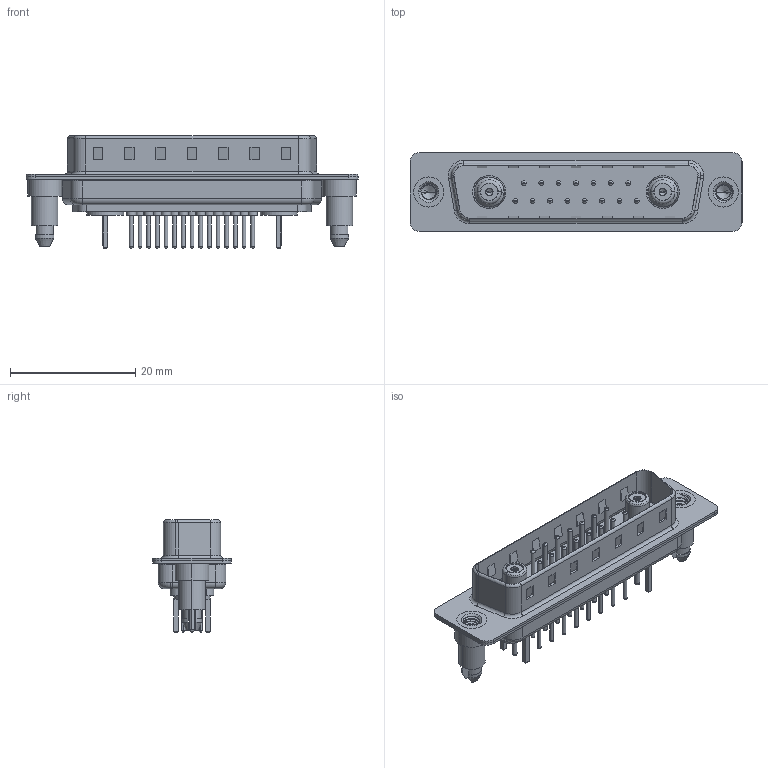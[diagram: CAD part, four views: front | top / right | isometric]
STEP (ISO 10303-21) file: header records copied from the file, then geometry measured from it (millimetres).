
FILE_DESCRIPTION (( 'STEP AP203' ), '1' );
FILE_NAME ('627-17W2224-7TD.STEP', '2019-05-27T21:48:21', ( '' ), ( '' ), 'SwSTEP 2.0', 'SolidWorks 2016', '' );
FILE_SCHEMA (( 'CONFIG_CONTROL_DESIGN' ));
Length unit declared in the file: millimetre
Products named in the file (14): Insulator Socket; 627Combo Shell Front_25 Contacts; 627Combo Threaded Boardlock_D; 627-17W2224-7TD; 627Combo Housing_17W2; Locking Collar; 627Combo Threaded Boardlock_5; 627Combo Contact Row 2_24; Co-Ax Jack Assy_S; 627Combo Contact Row 1_24; Insulator Socket 2; Co-Ax Jack_Straight PC Tail; Socket_Str; 627Combo Shell Rear_25 Contacts
Assembly tree (27 placements, depth 3):
  627-17W2224-7TD
    627Combo Housing_17W2
    627Combo Shell Rear_25 Contacts
    627Combo Shell Front_25 Contacts
    627Combo Threaded Boardlock_D
    Co-Ax Jack Assy_S  x2
      Co-Ax Jack_Straight PC Tail
      Insulator Socket
      Insulator Socket 2
      Locking Collar
      Socket_Str
    627Combo Threaded Boardlock_5
    627Combo Contact Row 1_24  x7
    627Combo Contact Row 2_24  x8
Bounding box: 53 x 12.6 x 17.9 mm (x, y, z)
Volume: 2896.4 mm3; surface area: 7933.7 mm2
Topology: 30 solids, 30 shells, 1211 faces, 2717 edges, 1672 vertices
Faces by surface type: cylinder 481, plane 386, torus 298, cone 31, bspline 11, sphere 4
Entity records: 26993 total; most frequent: CARTESIAN_POINT 7733, DIRECTION 3836, ORIENTED_EDGE 3484, EDGE_CURVE 1742, AXIS2_PLACEMENT_3D 1493, VERTEX_POINT 1108, EDGE_LOOP 878, VECTOR 850
